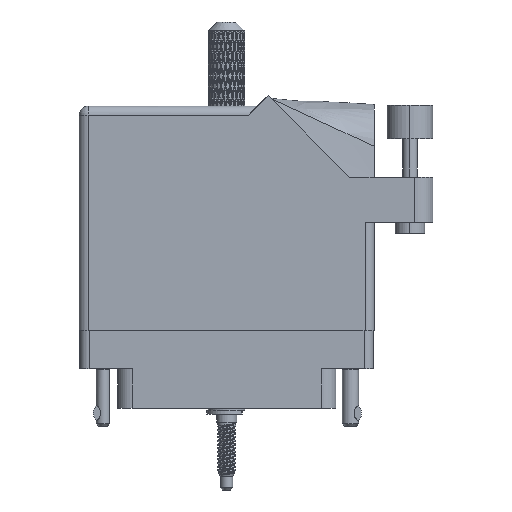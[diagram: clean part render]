
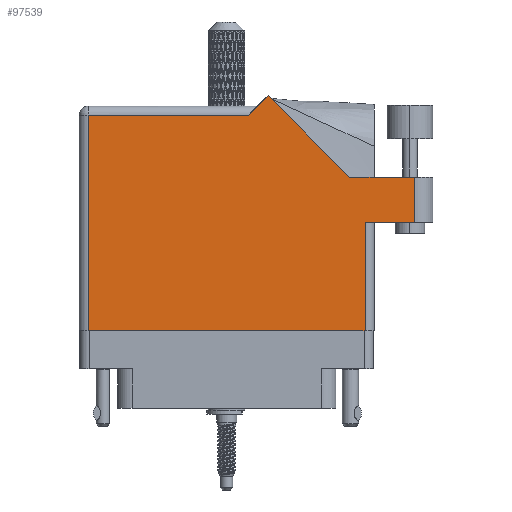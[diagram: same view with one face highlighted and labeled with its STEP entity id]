
A CAD part, front view. The second image highlights one B-rep face of the part: STEP entity #97539.
In plain terms, the highlighted face is planar.
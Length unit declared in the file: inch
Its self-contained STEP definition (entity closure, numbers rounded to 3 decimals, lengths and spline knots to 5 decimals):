
#1182 = CARTESIAN_POINT ( 'NONE',  ( 2.285, 1.044, 0. ) ) ;
#1440 = ORIENTED_EDGE ( 'NONE', *, *, #60360, .T. ) ;
#4393 = EDGE_CURVE ( 'NONE', #51367, #27836, #38812, .T. ) ;
#4688 = DIRECTION ( 'NONE',  ( -0.707, -0.707, 0. ) ) ;
#7175 = CARTESIAN_POINT ( 'NONE',  ( 1.28771, 1.60071, 0. ) ) ;
#8696 = EDGE_CURVE ( 'NONE', #26896, #30525, #21936, .T. ) ;
#10031 = LINE ( 'NONE', #75740, #100746 ) ;
#13961 = CARTESIAN_POINT ( 'NONE',  ( 2.41, 1.044, 0. ) ) ;
#14059 = VERTEX_POINT ( 'NONE', #67667 ) ;
#15348 = CARTESIAN_POINT ( 'NONE',  ( 0.062, 0., 0. ) ) ;
#19410 = CARTESIAN_POINT ( 'NONE',  ( 1.84442, 1.044, 0. ) ) ;
#20856 = VERTEX_POINT ( 'NONE', #104709 ) ;
#21468 = VERTEX_POINT ( 'NONE', #63233 ) ;
#21580 = EDGE_CURVE ( 'NONE', #72859, #51367, #52867, .T. ) ;
#21936 = LINE ( 'NONE', #92112, #86600 ) ;
#23122 = ORIENTED_EDGE ( 'NONE', *, *, #102256, .T. ) ;
#25578 = VECTOR ( 'NONE', #28838, 39.37008 ) ;
#26896 = VERTEX_POINT ( 'NONE', #91954 ) ;
#27322 = EDGE_CURVE ( 'NONE', #98098, #21468, #36874, .T. ) ;
#27836 = VERTEX_POINT ( 'NONE', #7175 ) ;
#28838 = DIRECTION ( 'NONE',  ( 1., 0., 0. ) ) ;
#29865 = LINE ( 'NONE', #47548, #56012 ) ;
#30162 = EDGE_CURVE ( 'NONE', #21468, #14059, #48936, .T. ) ;
#30525 = VERTEX_POINT ( 'NONE', #46384 ) ;
#30654 = DIRECTION ( 'NONE',  ( 0., 1., 0. ) ) ;
#30790 = CARTESIAN_POINT ( 'NONE',  ( 2.285, 1.044, 0. ) ) ;
#33902 = EDGE_CURVE ( 'NONE', #27836, #20856, #10031, .T. ) ;
#34842 = VECTOR ( 'NONE', #44074, 39.37008 ) ;
#36874 = LINE ( 'NONE', #15348, #111093 ) ;
#38812 = LINE ( 'NONE', #19410, #34842 ) ;
#44074 = DIRECTION ( 'NONE',  ( -0.707, 0.707, 0. ) ) ;
#45775 = CARTESIAN_POINT ( 'NONE',  ( 0., 0., 0. ) ) ;
#46384 = CARTESIAN_POINT ( 'NONE',  ( 2.285, 0.737, 0. ) ) ;
#47548 = CARTESIAN_POINT ( 'NONE',  ( 1.948, 0.737, 0. ) ) ;
#47976 = ORIENTED_EDGE ( 'NONE', *, *, #8696, .T. ) ;
#48780 = PLANE ( 'NONE',  #106665 ) ;
#48936 = LINE ( 'NONE', #45775, #25578 ) ;
#51367 = VERTEX_POINT ( 'NONE', #76402 ) ;
#52867 = LINE ( 'NONE', #13961, #91364 ) ;
#56012 = VECTOR ( 'NONE', #30654, 39.37008 ) ;
#56182 = ORIENTED_EDGE ( 'NONE', *, *, #4393, .T. ) ;
#57628 = DIRECTION ( 'NONE',  ( -1., 0., 0. ) ) ;
#57910 = CARTESIAN_POINT ( 'NONE',  ( 0.062, 1.468, 0. ) ) ;
#57957 = EDGE_CURVE ( 'NONE', #30525, #72859, #106859, .T. ) ;
#58093 = DIRECTION ( 'NONE',  ( 0., 1., 0. ) ) ;
#58433 = VECTOR ( 'NONE', #97421, 39.37008 ) ;
#60360 = EDGE_CURVE ( 'NONE', #20856, #98098, #81709, .T. ) ;
#62964 = ORIENTED_EDGE ( 'NONE', *, *, #30162, .T. ) ;
#63233 = CARTESIAN_POINT ( 'NONE',  ( 0.062, 0., 0. ) ) ;
#65309 = CARTESIAN_POINT ( 'NONE',  ( 0., 1.53, 0. ) ) ;
#67667 = CARTESIAN_POINT ( 'NONE',  ( 1.948, 0., 0. ) ) ;
#67954 = FACE_OUTER_BOUND ( 'NONE', #109982, .T. ) ;
#72859 = VERTEX_POINT ( 'NONE', #1182 ) ;
#75740 = CARTESIAN_POINT ( 'NONE',  ( 1.217, 1.53, 0. ) ) ;
#76402 = CARTESIAN_POINT ( 'NONE',  ( 1.84442, 1.044, 0. ) ) ;
#80533 = CARTESIAN_POINT ( 'NONE',  ( 0., 1.468, 0. ) ) ;
#81709 = LINE ( 'NONE', #80533, #58433 ) ;
#84714 = DIRECTION ( 'NONE',  ( -1., 0., 0. ) ) ;
#86600 = VECTOR ( 'NONE', #96379, 39.37008 ) ;
#87437 = ORIENTED_EDGE ( 'NONE', *, *, #57957, .T. ) ;
#89000 = ORIENTED_EDGE ( 'NONE', *, *, #21580, .T. ) ;
#91364 = VECTOR ( 'NONE', #84714, 39.37008 ) ;
#91954 = CARTESIAN_POINT ( 'NONE',  ( 1.948, 0.737, 0. ) ) ;
#92112 = CARTESIAN_POINT ( 'NONE',  ( 2.01, 0.737, 0. ) ) ;
#93255 = ORIENTED_EDGE ( 'NONE', *, *, #33902, .T. ) ;
#96379 = DIRECTION ( 'NONE',  ( 1., 0., 0. ) ) ;
#97421 = DIRECTION ( 'NONE',  ( -1., 0., 0. ) ) ;
#97539 = ADVANCED_FACE ( 'NONE', ( #67954 ), #48780, .F. ) ;
#98098 = VERTEX_POINT ( 'NONE', #57910 ) ;
#99991 = VECTOR ( 'NONE', #58093, 39.37008 ) ;
#100746 = VECTOR ( 'NONE', #4688, 39.37008 ) ;
#102217 = DIRECTION ( 'NONE',  ( 0., -1., 0. ) ) ;
#102256 = EDGE_CURVE ( 'NONE', #14059, #26896, #29865, .T. ) ;
#104709 = CARTESIAN_POINT ( 'NONE',  ( 1.155, 1.468, 0. ) ) ;
#106665 = AXIS2_PLACEMENT_3D ( 'NONE', #65309, #110224, #57628 ) ;
#106859 = LINE ( 'NONE', #30790, #99991 ) ;
#109982 = EDGE_LOOP ( 'NONE', ( #47976, #87437, #89000, #56182, #93255, #1440, #113253, #62964, #23122 ) ) ;
#110224 = DIRECTION ( 'NONE',  ( 0., 0., -1. ) ) ;
#111093 = VECTOR ( 'NONE', #102217, 39.37008 ) ;
#113253 = ORIENTED_EDGE ( 'NONE', *, *, #27322, .T. ) ;
